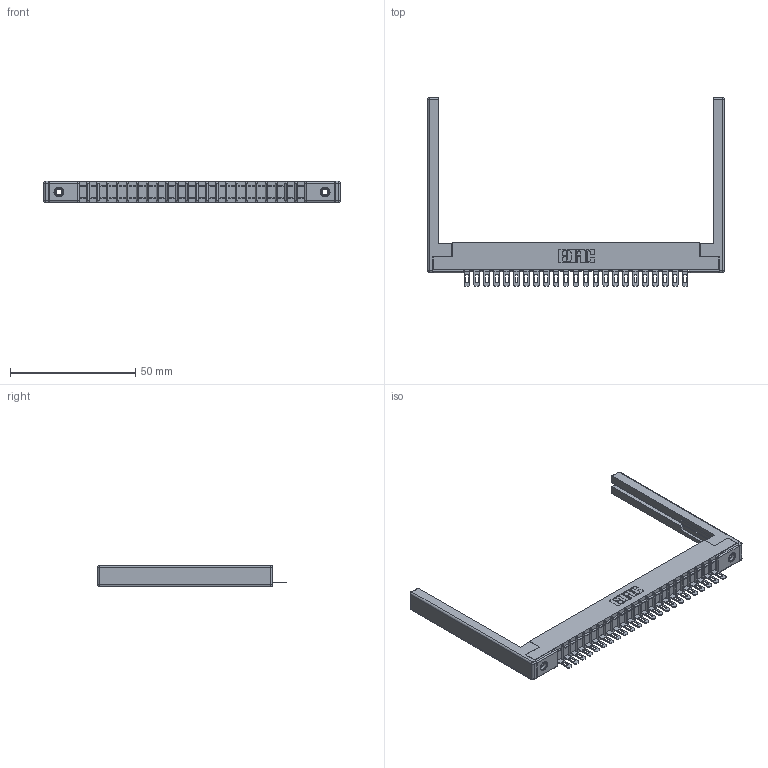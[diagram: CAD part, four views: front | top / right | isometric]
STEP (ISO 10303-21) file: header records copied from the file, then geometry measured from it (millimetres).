
FILE_DESCRIPTION (( 'STEP AP203' ), '1' );
FILE_NAME ('357-023-501-168.STEP', '2019-09-16T23:33:24', ( '' ), ( '' ), 'SwSTEP 2.0', 'SolidWorks 2016', '' );
FILE_SCHEMA (( 'CONFIG_CONTROL_DESIGN' ));
Length unit declared in the file: inch
Products named in the file (5): 345-250-001_345-250-001-102; 307-290-002_501; 307-220-068; 307 Part_.156 Dia Mounting Holes; 357-023-501-168
Assembly tree (28 placements, depth 2):
  357-023-501-168
    307 Part_.156 Dia Mounting Holes
    307-290-002_501  x23
    307-220-068  x2
    345-250-001_345-250-001-102  x2
Bounding box: 118.57 x 75.39 x 8.71 mm (x, y, z)
Volume: 12406.9 mm3; surface area: 18505.4 mm2
Topology: 28 solids, 28 shells, 2044 faces, 6187 edges, 4038 vertices
Faces by surface type: plane 1170, cylinder 802, sphere 56, cone 12, torus 4
Entity records: 25613 total; most frequent: CARTESIAN_POINT 4281, ORIENTED_EDGE 4260, DIRECTION 4190, EDGE_CURVE 2130, VECTOR 1616, LINE 1616, VERTEX_POINT 1378, AXIS2_PLACEMENT_3D 1287
